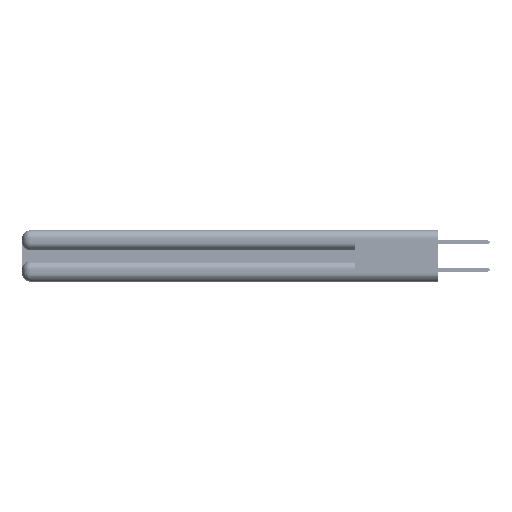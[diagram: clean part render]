
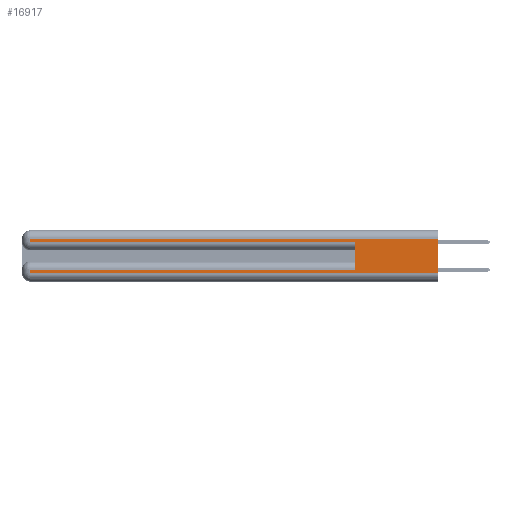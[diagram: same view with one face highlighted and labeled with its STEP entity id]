
A CAD part, left-side view. The second image highlights one B-rep face of the part: STEP entity #16917.
In plain terms, the highlighted planar face has unit normal (-1, 0, 0).
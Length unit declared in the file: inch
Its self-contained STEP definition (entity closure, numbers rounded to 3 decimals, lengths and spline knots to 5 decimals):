
#325 = CARTESIAN_POINT ( 'NONE',  ( 0., 0., 0.37 ) ) ;
#1104 = CARTESIAN_POINT ( 'NONE',  ( 0., 2.94, 0.31 ) ) ;
#2325 = LINE ( 'NONE', #12405, #19814 ) ;
#2350 = DIRECTION ( 'NONE',  ( 0., 0., -1. ) ) ;
#5908 = DIRECTION ( 'NONE',  ( 0., 0., -1. ) ) ;
#6585 = VERTEX_POINT ( 'NONE', #11990 ) ;
#6664 = CARTESIAN_POINT ( 'NONE',  ( 0., 0., 0.31 ) ) ;
#7238 = CARTESIAN_POINT ( 'NONE',  ( 0., 2.94, 0.085 ) ) ;
#7905 = CARTESIAN_POINT ( 'NONE',  ( 0., 0.6, 0.085 ) ) ;
#8335 = VERTEX_POINT ( 'NONE', #20854 ) ;
#8818 = EDGE_LOOP ( 'NONE', ( #11583, #15291, #47196, #50161, #21638, #51494, #19414, #14825 ) ) ;
#9662 = VECTOR ( 'NONE', #23360, 39.37008 ) ;
#9725 = VERTEX_POINT ( 'NONE', #46309 ) ;
#10623 = LINE ( 'NONE', #45025, #20354 ) ;
#11096 = CARTESIAN_POINT ( 'NONE',  ( 0., 2.94, 0.06 ) ) ;
#11583 = ORIENTED_EDGE ( 'NONE', *, *, #34640, .F. ) ;
#11990 = CARTESIAN_POINT ( 'NONE',  ( 0., 2.94, 0.285 ) ) ;
#12405 = CARTESIAN_POINT ( 'NONE',  ( 0., 0.6, 0.145 ) ) ;
#13120 = CARTESIAN_POINT ( 'NONE',  ( 0., 0., 0.085 ) ) ;
#13293 = VERTEX_POINT ( 'NONE', #7905 ) ;
#14234 = VERTEX_POINT ( 'NONE', #11096 ) ;
#14825 = ORIENTED_EDGE ( 'NONE', *, *, #30857, .T. ) ;
#15171 = VECTOR ( 'NONE', #2350, 39.37008 ) ;
#15291 = ORIENTED_EDGE ( 'NONE', *, *, #38394, .T. ) ;
#16917 = ADVANCED_FACE ( 'NONE', ( #21473 ), #42295, .F. ) ;
#19260 = CARTESIAN_POINT ( 'NONE',  ( 0., 0., 0.31 ) ) ;
#19414 = ORIENTED_EDGE ( 'NONE', *, *, #36278, .T. ) ;
#19814 = VECTOR ( 'NONE', #37110, 39.37008 ) ;
#20309 = LINE ( 'NONE', #13120, #44364 ) ;
#20354 = VECTOR ( 'NONE', #28098, 39.37008 ) ;
#20695 = VECTOR ( 'NONE', #35704, 39.37008 ) ;
#20854 = CARTESIAN_POINT ( 'NONE',  ( 0., 0., 0.06 ) ) ;
#21282 = VERTEX_POINT ( 'NONE', #19260 ) ;
#21455 = AXIS2_PLACEMENT_3D ( 'NONE', #21593, #50686, #34488 ) ;
#21473 = FACE_OUTER_BOUND ( 'NONE', #8818, .T. ) ;
#21593 = CARTESIAN_POINT ( 'NONE',  ( 0., 0., 0.37 ) ) ;
#21638 = ORIENTED_EDGE ( 'NONE', *, *, #26439, .F. ) ;
#23360 = DIRECTION ( 'NONE',  ( 0., -1., 0. ) ) ;
#26183 = LINE ( 'NONE', #26997, #15171 ) ;
#26439 = EDGE_CURVE ( 'NONE', #13293, #9725, #2325, .T. ) ;
#26997 = CARTESIAN_POINT ( 'NONE',  ( 0., 2.94, 0.37 ) ) ;
#27166 = LINE ( 'NONE', #6664, #20695 ) ;
#28098 = DIRECTION ( 'NONE',  ( 0., -1., 0. ) ) ;
#30857 = EDGE_CURVE ( 'NONE', #14234, #8335, #38903, .T. ) ;
#32230 = VECTOR ( 'NONE', #45537, 39.37008 ) ;
#34488 = DIRECTION ( 'NONE',  ( 0., 0., -1. ) ) ;
#34640 = EDGE_CURVE ( 'NONE', #21282, #8335, #40638, .T. ) ;
#35362 = CARTESIAN_POINT ( 'NONE',  ( 0., 0., 0.06 ) ) ;
#35704 = DIRECTION ( 'NONE',  ( 0., 1., 0. ) ) ;
#36278 = EDGE_CURVE ( 'NONE', #42918, #14234, #26183, .T. ) ;
#37110 = DIRECTION ( 'NONE',  ( 0., 0., 1. ) ) ;
#38394 = EDGE_CURVE ( 'NONE', #21282, #48554, #27166, .T. ) ;
#38859 = EDGE_CURVE ( 'NONE', #48554, #6585, #50389, .T. ) ;
#38903 = LINE ( 'NONE', #35362, #9662 ) ;
#39317 = VECTOR ( 'NONE', #5908, 39.37008 ) ;
#39895 = EDGE_CURVE ( 'NONE', #6585, #9725, #10623, .T. ) ;
#40638 = LINE ( 'NONE', #325, #32230 ) ;
#42295 = PLANE ( 'NONE',  #21455 ) ;
#42918 = VERTEX_POINT ( 'NONE', #7238 ) ;
#44364 = VECTOR ( 'NONE', #46536, 39.37008 ) ;
#45025 = CARTESIAN_POINT ( 'NONE',  ( 0., 0., 0.285 ) ) ;
#45537 = DIRECTION ( 'NONE',  ( 0., 0., -1. ) ) ;
#46309 = CARTESIAN_POINT ( 'NONE',  ( 0., 0.6, 0.285 ) ) ;
#46536 = DIRECTION ( 'NONE',  ( 0., 1., 0. ) ) ;
#47114 = CARTESIAN_POINT ( 'NONE',  ( 0., 2.94, 0.37 ) ) ;
#47196 = ORIENTED_EDGE ( 'NONE', *, *, #38859, .T. ) ;
#48554 = VERTEX_POINT ( 'NONE', #1104 ) ;
#50161 = ORIENTED_EDGE ( 'NONE', *, *, #39895, .T. ) ;
#50389 = LINE ( 'NONE', #47114, #39317 ) ;
#50577 = EDGE_CURVE ( 'NONE', #13293, #42918, #20309, .T. ) ;
#50686 = DIRECTION ( 'NONE',  ( 1., 0., 0. ) ) ;
#51494 = ORIENTED_EDGE ( 'NONE', *, *, #50577, .T. ) ;
